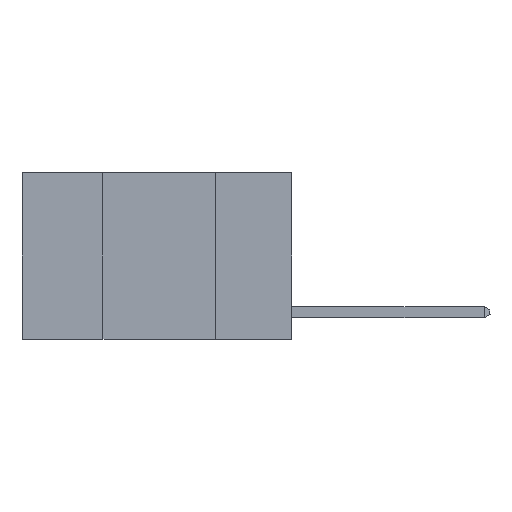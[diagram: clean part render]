
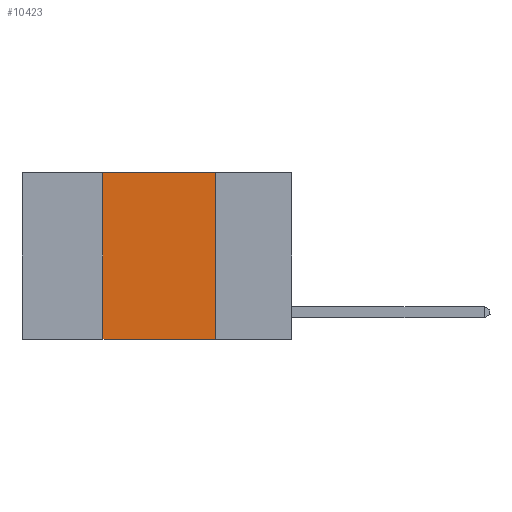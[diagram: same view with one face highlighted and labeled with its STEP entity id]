
A CAD part, left-side view. The second image highlights one B-rep face of the part: STEP entity #10423.
In plain terms, the highlighted planar face has unit normal (-1, 0, 0).
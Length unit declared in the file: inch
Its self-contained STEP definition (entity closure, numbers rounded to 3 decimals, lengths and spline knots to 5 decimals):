
#536 = DIRECTION ( 'NONE',  ( 0., 0., 1. ) ) ;
#578 = VERTEX_POINT ( 'NONE', #2903 ) ;
#839 = CARTESIAN_POINT ( 'NONE',  ( 0., 0.6, 0. ) ) ;
#1294 = EDGE_CURVE ( 'NONE', #3053, #578, #4108, .T. ) ;
#1385 = EDGE_CURVE ( 'NONE', #3053, #15110, #3381, .T. ) ;
#1423 = EDGE_CURVE ( 'NONE', #14986, #15110, #7142, .T. ) ;
#2103 = ORIENTED_EDGE ( 'NONE', *, *, #1423, .F. ) ;
#2148 = DIRECTION ( 'NONE',  ( 0., 0., -1. ) ) ;
#2518 = VECTOR ( 'NONE', #536, 39.37008 ) ;
#2903 = CARTESIAN_POINT ( 'NONE',  ( 0., 0.42, 0. ) ) ;
#3053 = VERTEX_POINT ( 'NONE', #10358 ) ;
#3381 = LINE ( 'NONE', #10684, #12835 ) ;
#3858 = DIRECTION ( 'NONE',  ( 0., 0., -1. ) ) ;
#4108 = LINE ( 'NONE', #14084, #2518 ) ;
#4562 = VECTOR ( 'NONE', #13173, 39.37008 ) ;
#4995 = CARTESIAN_POINT ( 'NONE',  ( 0., 0.6, 0. ) ) ;
#5950 = DIRECTION ( 'NONE',  ( 0., -1., 0. ) ) ;
#6070 = ORIENTED_EDGE ( 'NONE', *, *, #1385, .T. ) ;
#6188 = FACE_OUTER_BOUND ( 'NONE', #12149, .T. ) ;
#7142 = LINE ( 'NONE', #13191, #14907 ) ;
#9891 = AXIS2_PLACEMENT_3D ( 'NONE', #4995, #14889, #3858 ) ;
#10358 = CARTESIAN_POINT ( 'NONE',  ( 0., 0.42, -0.37 ) ) ;
#10423 = ADVANCED_FACE ( 'NONE', ( #6188 ), #11086, .F. ) ;
#10652 = CARTESIAN_POINT ( 'NONE',  ( 0., 0.17, -0.37 ) ) ;
#10684 = CARTESIAN_POINT ( 'NONE',  ( 0., 0.6, -0.37 ) ) ;
#11086 = PLANE ( 'NONE',  #9891 ) ;
#11535 = CARTESIAN_POINT ( 'NONE',  ( 0., 0.17, 0. ) ) ;
#11801 = LINE ( 'NONE', #839, #4562 ) ;
#12051 = ORIENTED_EDGE ( 'NONE', *, *, #1294, .F. ) ;
#12149 = EDGE_LOOP ( 'NONE', ( #2103, #12697, #12051, #6070 ) ) ;
#12697 = ORIENTED_EDGE ( 'NONE', *, *, #14683, .F. ) ;
#12835 = VECTOR ( 'NONE', #5950, 39.37008 ) ;
#13173 = DIRECTION ( 'NONE',  ( 0., -1., 0. ) ) ;
#13191 = CARTESIAN_POINT ( 'NONE',  ( 0., 0.17, 0. ) ) ;
#14084 = CARTESIAN_POINT ( 'NONE',  ( 0., 0.42, 0. ) ) ;
#14683 = EDGE_CURVE ( 'NONE', #578, #14986, #11801, .T. ) ;
#14889 = DIRECTION ( 'NONE',  ( 1., 0., 0. ) ) ;
#14907 = VECTOR ( 'NONE', #2148, 39.37008 ) ;
#14986 = VERTEX_POINT ( 'NONE', #11535 ) ;
#15110 = VERTEX_POINT ( 'NONE', #10652 ) ;
